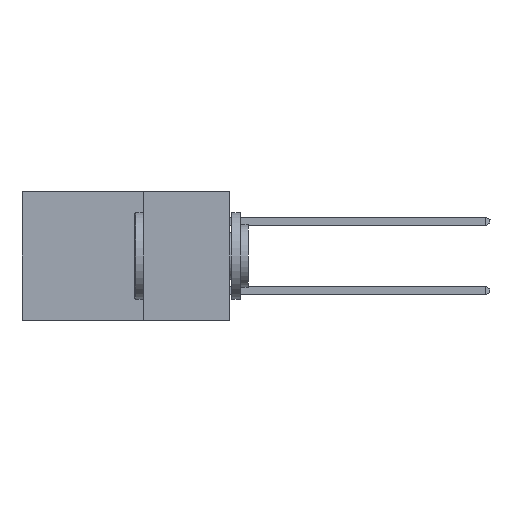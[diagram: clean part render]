
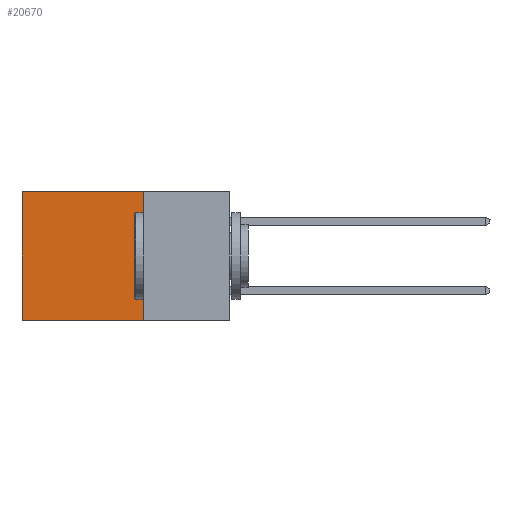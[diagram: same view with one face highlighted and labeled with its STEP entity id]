
A CAD part, left-side view. The second image highlights one B-rep face of the part: STEP entity #20670.
In plain terms, the highlighted planar face has unit normal (-1, 0, 0).
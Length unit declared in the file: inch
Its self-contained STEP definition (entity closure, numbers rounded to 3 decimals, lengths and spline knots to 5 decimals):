
#3472 = DIRECTION ( 'NONE',  ( 0., 0., -1. ) ) ;
#4589 = CARTESIAN_POINT ( 'NONE',  ( 0.298, 0.25, -0.37 ) ) ;
#4833 = VERTEX_POINT ( 'NONE', #11210 ) ;
#6311 = CARTESIAN_POINT ( 'NONE',  ( 0.298, 0.6, 0. ) ) ;
#6507 = ORIENTED_EDGE ( 'NONE', *, *, #26017, .T. ) ;
#7271 = CARTESIAN_POINT ( 'NONE',  ( 0.298, 0.25, 0. ) ) ;
#7865 = CARTESIAN_POINT ( 'NONE',  ( 0.298, 0.25, 0. ) ) ;
#8278 = EDGE_CURVE ( 'NONE', #22353, #15541, #19178, .T. ) ;
#8819 = ORIENTED_EDGE ( 'NONE', *, *, #8278, .F. ) ;
#10207 = DIRECTION ( 'NONE',  ( 0., 0., -1. ) ) ;
#10387 = DIRECTION ( 'NONE',  ( 1., 0., 0. ) ) ;
#11210 = CARTESIAN_POINT ( 'NONE',  ( 0.298, 0.25, 0. ) ) ;
#11944 = VECTOR ( 'NONE', #26200, 39.37008 ) ;
#12701 = VECTOR ( 'NONE', #22930, 39.37008 ) ;
#13422 = LINE ( 'NONE', #7865, #14758 ) ;
#14688 = ORIENTED_EDGE ( 'NONE', *, *, #18243, .T. ) ;
#14758 = VECTOR ( 'NONE', #22376, 39.37008 ) ;
#14872 = CARTESIAN_POINT ( 'NONE',  ( 0.298, 0.25, -0.37 ) ) ;
#15541 = VERTEX_POINT ( 'NONE', #23299 ) ;
#16611 = CARTESIAN_POINT ( 'NONE',  ( 0.298, 0.25, 0. ) ) ;
#17907 = VECTOR ( 'NONE', #3472, 39.37008 ) ;
#18041 = VERTEX_POINT ( 'NONE', #6311 ) ;
#18243 = EDGE_CURVE ( 'NONE', #18041, #15541, #24257, .T. ) ;
#19178 = LINE ( 'NONE', #14872, #11944 ) ;
#19531 = LINE ( 'NONE', #7271, #17907 ) ;
#19995 = EDGE_LOOP ( 'NONE', ( #14688, #8819, #21884, #6507 ) ) ;
#20670 = ADVANCED_FACE ( 'NONE', ( #26478 ), #23022, .F. ) ;
#21734 = AXIS2_PLACEMENT_3D ( 'NONE', #16611, #10387, #10207 ) ;
#21884 = ORIENTED_EDGE ( 'NONE', *, *, #22396, .F. ) ;
#22353 = VERTEX_POINT ( 'NONE', #4589 ) ;
#22376 = DIRECTION ( 'NONE',  ( 0., 1., 0. ) ) ;
#22396 = EDGE_CURVE ( 'NONE', #4833, #22353, #19531, .T. ) ;
#22930 = DIRECTION ( 'NONE',  ( 0., 0., -1. ) ) ;
#23022 = PLANE ( 'NONE',  #21734 ) ;
#23299 = CARTESIAN_POINT ( 'NONE',  ( 0.298, 0.6, -0.37 ) ) ;
#24257 = LINE ( 'NONE', #27309, #12701 ) ;
#26017 = EDGE_CURVE ( 'NONE', #4833, #18041, #13422, .T. ) ;
#26200 = DIRECTION ( 'NONE',  ( 0., 1., 0. ) ) ;
#26478 = FACE_OUTER_BOUND ( 'NONE', #19995, .T. ) ;
#27309 = CARTESIAN_POINT ( 'NONE',  ( 0.298, 0.6, 0. ) ) ;
